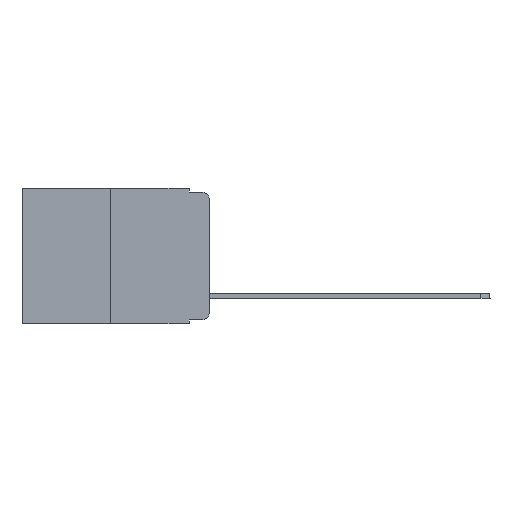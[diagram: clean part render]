
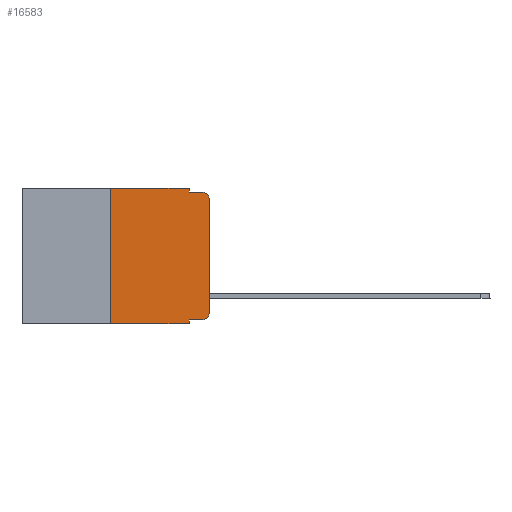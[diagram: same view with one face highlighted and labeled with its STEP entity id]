
A CAD part, left-side view. The second image highlights one B-rep face of the part: STEP entity #16583.
In plain terms, the highlighted planar face has unit normal (-1, 0, 0).
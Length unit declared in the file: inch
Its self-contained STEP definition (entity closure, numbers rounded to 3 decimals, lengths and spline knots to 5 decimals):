
#528 = EDGE_CURVE ( 'NONE', #5707, #3373, #1000, .T. ) ;
#750 = EDGE_CURVE ( 'NONE', #5707, #18732, #7621, .T. ) ;
#798 = CARTESIAN_POINT ( 'NONE',  ( 0., 0.02, -0.01 ) ) ;
#839 = EDGE_CURVE ( 'NONE', #8818, #3458, #23017, .T. ) ;
#1000 = LINE ( 'NONE', #11569, #19533 ) ;
#1420 = EDGE_CURVE ( 'NONE', #20044, #8818, #3652, .T. ) ;
#1644 = DIRECTION ( 'NONE',  ( 0., 0., 1. ) ) ;
#1798 = ORIENTED_EDGE ( 'NONE', *, *, #1420, .T. ) ;
#2106 = CARTESIAN_POINT ( 'NONE',  ( 0., 0.051, -0.343 ) ) ;
#2232 = CARTESIAN_POINT ( 'NONE',  ( 0., 0.25, 0. ) ) ;
#2933 = ORIENTED_EDGE ( 'NONE', *, *, #10483, .T. ) ;
#3085 = DIRECTION ( 'NONE',  ( 1., 0., 0. ) ) ;
#3373 = VERTEX_POINT ( 'NONE', #2232 ) ;
#3458 = VERTEX_POINT ( 'NONE', #22046 ) ;
#3471 = CARTESIAN_POINT ( 'NONE',  ( 0., 0.02, -0.03 ) ) ;
#3599 = CARTESIAN_POINT ( 'NONE',  ( 0., 0.02, -0.313 ) ) ;
#3618 = VERTEX_POINT ( 'NONE', #6740 ) ;
#3641 = AXIS2_PLACEMENT_3D ( 'NONE', #4932, #3085, #15650 ) ;
#3652 = LINE ( 'NONE', #9274, #8469 ) ;
#3669 = DIRECTION ( 'NONE',  ( -1., 0., 0. ) ) ;
#3671 = VECTOR ( 'NONE', #13876, 39.37008 ) ;
#3962 = EDGE_LOOP ( 'NONE', ( #2933, #15075, #14054, #21705, #7969, #8485, #14443, #18763, #1798, #19920 ) ) ;
#3993 = AXIS2_PLACEMENT_3D ( 'NONE', #3599, #3669, #7148 ) ;
#4548 = VECTOR ( 'NONE', #10398, 39.37008 ) ;
#4932 = CARTESIAN_POINT ( 'NONE',  ( 0., 0.473, 0. ) ) ;
#5667 = LINE ( 'NONE', #5781, #22193 ) ;
#5707 = VERTEX_POINT ( 'NONE', #13410 ) ;
#5721 = AXIS2_PLACEMENT_3D ( 'NONE', #3471, #17830, #15797 ) ;
#5781 = CARTESIAN_POINT ( 'NONE',  ( 0., 0.051, 0. ) ) ;
#6623 = CARTESIAN_POINT ( 'NONE',  ( 0., 0., -0.03 ) ) ;
#6645 = VERTEX_POINT ( 'NONE', #15364 ) ;
#6711 = CARTESIAN_POINT ( 'NONE',  ( 0., 0.473, 0. ) ) ;
#6740 = CARTESIAN_POINT ( 'NONE',  ( 0., 0.051, 0. ) ) ;
#7148 = DIRECTION ( 'NONE',  ( 0., 0., -1. ) ) ;
#7621 = LINE ( 'NONE', #8567, #3671 ) ;
#7712 = CARTESIAN_POINT ( 'NONE',  ( 0., 0.02, -0.333 ) ) ;
#7717 = EDGE_CURVE ( 'NONE', #6645, #8011, #12253, .T. ) ;
#7926 = VECTOR ( 'NONE', #1644, 39.37008 ) ;
#7969 = ORIENTED_EDGE ( 'NONE', *, *, #12956, .F. ) ;
#8011 = VERTEX_POINT ( 'NONE', #798 ) ;
#8469 = VECTOR ( 'NONE', #14663, 39.37008 ) ;
#8485 = ORIENTED_EDGE ( 'NONE', *, *, #528, .F. ) ;
#8567 = CARTESIAN_POINT ( 'NONE',  ( 0., 0.473, -0.343 ) ) ;
#8818 = VERTEX_POINT ( 'NONE', #7712 ) ;
#8820 = CARTESIAN_POINT ( 'NONE',  ( 0., 0.051, -0.333 ) ) ;
#9274 = CARTESIAN_POINT ( 'NONE',  ( 0., 0.051, -0.333 ) ) ;
#10342 = EDGE_CURVE ( 'NONE', #20044, #18732, #5667, .T. ) ;
#10398 = DIRECTION ( 'NONE',  ( 0., 0., -1. ) ) ;
#10483 = EDGE_CURVE ( 'NONE', #3458, #17250, #16039, .T. ) ;
#10999 = CIRCLE ( 'NONE', #5721, 0.02 ) ;
#11339 = VECTOR ( 'NONE', #18055, 39.37008 ) ;
#11569 = CARTESIAN_POINT ( 'NONE',  ( 0., 0.25, 0. ) ) ;
#11719 = FACE_OUTER_BOUND ( 'NONE', #3962, .T. ) ;
#11999 = CARTESIAN_POINT ( 'NONE',  ( 0., 0.051, -0.01 ) ) ;
#12253 = LINE ( 'NONE', #11999, #23165 ) ;
#12956 = EDGE_CURVE ( 'NONE', #3373, #3618, #14456, .T. ) ;
#13406 = DIRECTION ( 'NONE',  ( 0., 0., 1. ) ) ;
#13410 = CARTESIAN_POINT ( 'NONE',  ( 0., 0.25, -0.343 ) ) ;
#13595 = EDGE_CURVE ( 'NONE', #17250, #8011, #10999, .T. ) ;
#13876 = DIRECTION ( 'NONE',  ( 0., -1., 0. ) ) ;
#14054 = ORIENTED_EDGE ( 'NONE', *, *, #7717, .F. ) ;
#14443 = ORIENTED_EDGE ( 'NONE', *, *, #750, .T. ) ;
#14456 = LINE ( 'NONE', #6711, #11339 ) ;
#14616 = EDGE_CURVE ( 'NONE', #3618, #6645, #15182, .T. ) ;
#14663 = DIRECTION ( 'NONE',  ( 0., -1., 0. ) ) ;
#15075 = ORIENTED_EDGE ( 'NONE', *, *, #13595, .T. ) ;
#15182 = LINE ( 'NONE', #15739, #4548 ) ;
#15364 = CARTESIAN_POINT ( 'NONE',  ( 0., 0.051, -0.01 ) ) ;
#15650 = DIRECTION ( 'NONE',  ( 0., 0., -1. ) ) ;
#15739 = CARTESIAN_POINT ( 'NONE',  ( 0., 0.051, 0. ) ) ;
#15797 = DIRECTION ( 'NONE',  ( 0., 0., -1. ) ) ;
#16039 = LINE ( 'NONE', #21329, #7926 ) ;
#16583 = ADVANCED_FACE ( 'NONE', ( #11719 ), #21182, .F. ) ;
#17250 = VERTEX_POINT ( 'NONE', #6623 ) ;
#17374 = DIRECTION ( 'NONE',  ( 0., -1., 0. ) ) ;
#17830 = DIRECTION ( 'NONE',  ( -1., 0., 0. ) ) ;
#18055 = DIRECTION ( 'NONE',  ( 0., -1., 0. ) ) ;
#18332 = DIRECTION ( 'NONE',  ( 0., 0., -1. ) ) ;
#18732 = VERTEX_POINT ( 'NONE', #2106 ) ;
#18763 = ORIENTED_EDGE ( 'NONE', *, *, #10342, .F. ) ;
#19533 = VECTOR ( 'NONE', #13406, 39.37008 ) ;
#19920 = ORIENTED_EDGE ( 'NONE', *, *, #839, .T. ) ;
#20044 = VERTEX_POINT ( 'NONE', #8820 ) ;
#21182 = PLANE ( 'NONE',  #3641 ) ;
#21329 = CARTESIAN_POINT ( 'NONE',  ( 0., 0., 0. ) ) ;
#21705 = ORIENTED_EDGE ( 'NONE', *, *, #14616, .F. ) ;
#22046 = CARTESIAN_POINT ( 'NONE',  ( 0., 0., -0.313 ) ) ;
#22193 = VECTOR ( 'NONE', #18332, 39.37008 ) ;
#23017 = CIRCLE ( 'NONE', #3993, 0.02 ) ;
#23165 = VECTOR ( 'NONE', #17374, 39.37008 ) ;
